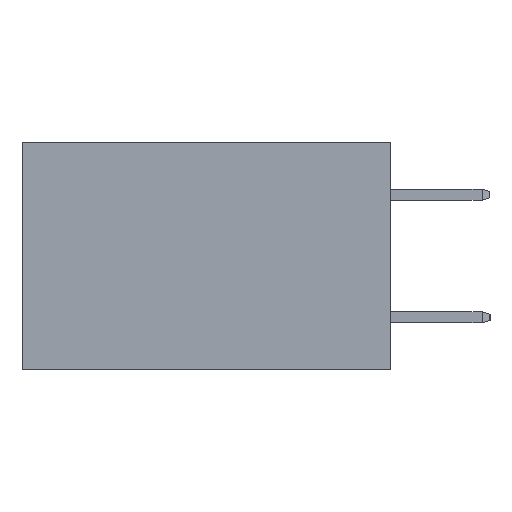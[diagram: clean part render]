
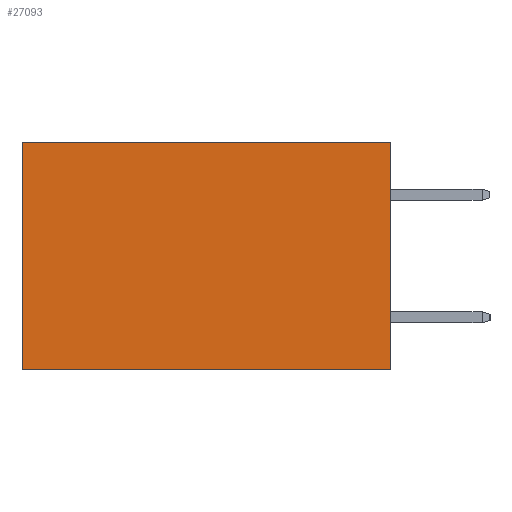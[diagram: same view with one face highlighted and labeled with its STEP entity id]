
A CAD part, left-side view. The second image highlights one B-rep face of the part: STEP entity #27093.
In plain terms, the highlighted planar face has unit normal (-1, 0, 0).
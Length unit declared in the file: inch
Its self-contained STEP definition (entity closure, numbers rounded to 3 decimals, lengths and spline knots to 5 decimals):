
#101 = VECTOR ( 'NONE', #7677, 39.37008 ) ;
#2349 = CARTESIAN_POINT ( 'NONE',  ( 0.2875, 0.6, -0.37 ) ) ;
#2708 = PLANE ( 'NONE',  #34488 ) ;
#4377 = CARTESIAN_POINT ( 'NONE',  ( 0.2875, 0., -0.37 ) ) ;
#4575 = VERTEX_POINT ( 'NONE', #19830 ) ;
#4688 = CARTESIAN_POINT ( 'NONE',  ( 0.2875, 0., 0. ) ) ;
#6914 = CARTESIAN_POINT ( 'NONE',  ( 0.2875, 0.6, 0. ) ) ;
#6959 = LINE ( 'NONE', #13118, #26040 ) ;
#7509 = CARTESIAN_POINT ( 'NONE',  ( 0.2875, 0.6, 0. ) ) ;
#7677 = DIRECTION ( 'NONE',  ( 0., 1., 0. ) ) ;
#7975 = VECTOR ( 'NONE', #8054, 39.37008 ) ;
#8054 = DIRECTION ( 'NONE',  ( 0., 0., -1. ) ) ;
#10793 = ORIENTED_EDGE ( 'NONE', *, *, #23914, .T. ) ;
#12066 = LINE ( 'NONE', #14255, #32838 ) ;
#13118 = CARTESIAN_POINT ( 'NONE',  ( 0.2875, 0., 0. ) ) ;
#13743 = DIRECTION ( 'NONE',  ( 0., 0., -1. ) ) ;
#13783 = EDGE_CURVE ( 'NONE', #4575, #26586, #6959, .T. ) ;
#14255 = CARTESIAN_POINT ( 'NONE',  ( 0.2875, 0., 0. ) ) ;
#15846 = LINE ( 'NONE', #7509, #7975 ) ;
#16449 = VERTEX_POINT ( 'NONE', #2349 ) ;
#19830 = CARTESIAN_POINT ( 'NONE',  ( 0.2875, 0., 0. ) ) ;
#21436 = LINE ( 'NONE', #32502, #101 ) ;
#22735 = ORIENTED_EDGE ( 'NONE', *, *, #23512, .F. ) ;
#22882 = VERTEX_POINT ( 'NONE', #4377 ) ;
#23512 = EDGE_CURVE ( 'NONE', #4575, #22882, #12066, .T. ) ;
#23914 = EDGE_CURVE ( 'NONE', #26586, #16449, #15846, .T. ) ;
#25103 = DIRECTION ( 'NONE',  ( 0., 0., -1. ) ) ;
#26040 = VECTOR ( 'NONE', #34332, 39.37008 ) ;
#26586 = VERTEX_POINT ( 'NONE', #6914 ) ;
#27093 = ADVANCED_FACE ( 'NONE', ( #27512 ), #2708, .F. ) ;
#27512 = FACE_OUTER_BOUND ( 'NONE', #32810, .T. ) ;
#29022 = ORIENTED_EDGE ( 'NONE', *, *, #34548, .F. ) ;
#29857 = DIRECTION ( 'NONE',  ( 1., 0., 0. ) ) ;
#30337 = ORIENTED_EDGE ( 'NONE', *, *, #13783, .T. ) ;
#32502 = CARTESIAN_POINT ( 'NONE',  ( 0.2875, 0., -0.37 ) ) ;
#32810 = EDGE_LOOP ( 'NONE', ( #10793, #29022, #22735, #30337 ) ) ;
#32838 = VECTOR ( 'NONE', #25103, 39.37008 ) ;
#34332 = DIRECTION ( 'NONE',  ( 0., 1., 0. ) ) ;
#34488 = AXIS2_PLACEMENT_3D ( 'NONE', #4688, #29857, #13743 ) ;
#34548 = EDGE_CURVE ( 'NONE', #22882, #16449, #21436, .T. ) ;
